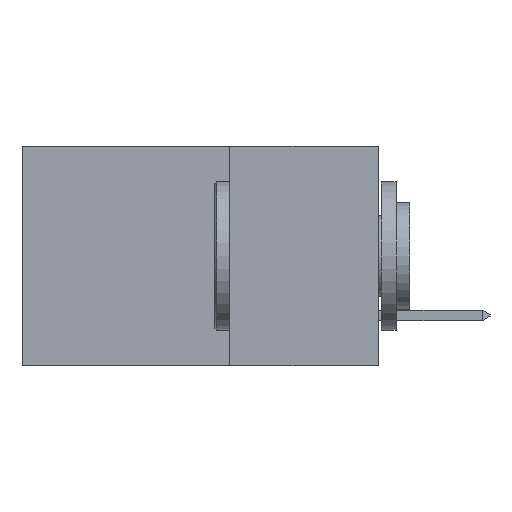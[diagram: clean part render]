
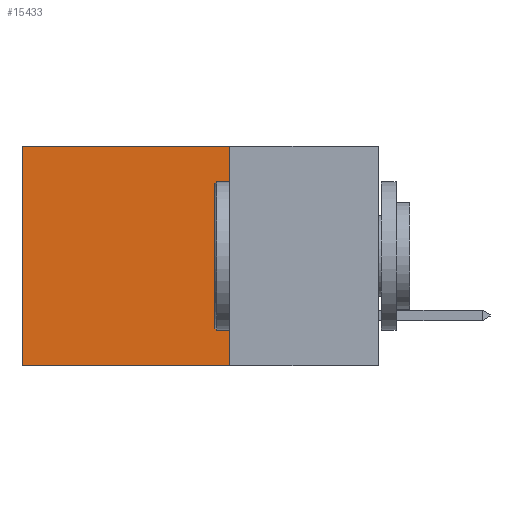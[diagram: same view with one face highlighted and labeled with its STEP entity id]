
A CAD part, left-side view. The second image highlights one B-rep face of the part: STEP entity #15433.
In plain terms, the highlighted planar face has unit normal (-1, 0, 0).
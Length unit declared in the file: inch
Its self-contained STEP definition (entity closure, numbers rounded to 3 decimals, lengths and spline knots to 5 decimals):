
#584 = ORIENTED_EDGE ( 'NONE', *, *, #5645, .F. ) ;
#1097 = FACE_OUTER_BOUND ( 'NONE', #2880, .T. ) ;
#1287 = ORIENTED_EDGE ( 'NONE', *, *, #19993, .F. ) ;
#1569 = LINE ( 'NONE', #4928, #19775 ) ;
#2152 = LINE ( 'NONE', #17924, #16239 ) ;
#2165 = CARTESIAN_POINT ( 'NONE',  ( 0.298, 0.25, 0. ) ) ;
#2408 = VECTOR ( 'NONE', #8987, 39.37008 ) ;
#2507 = ORIENTED_EDGE ( 'NONE', *, *, #7538, .T. ) ;
#2880 = EDGE_LOOP ( 'NONE', ( #13797, #584, #1287, #2507 ) ) ;
#3808 = PLANE ( 'NONE',  #9138 ) ;
#3880 = DIRECTION ( 'NONE',  ( 0., 0., -1. ) ) ;
#4108 = DIRECTION ( 'NONE',  ( 0., 1., 0. ) ) ;
#4928 = CARTESIAN_POINT ( 'NONE',  ( 0.298, 0.25, 0. ) ) ;
#5219 = VECTOR ( 'NONE', #4108, 39.37008 ) ;
#5645 = EDGE_CURVE ( 'NONE', #12891, #8686, #14137, .T. ) ;
#7235 = CARTESIAN_POINT ( 'NONE',  ( 0.298, 0.6, -0.37 ) ) ;
#7538 = EDGE_CURVE ( 'NONE', #11624, #19012, #15942, .T. ) ;
#8686 = VERTEX_POINT ( 'NONE', #7235 ) ;
#8987 = DIRECTION ( 'NONE',  ( 0., 1., 0. ) ) ;
#9079 = CARTESIAN_POINT ( 'NONE',  ( 0.298, 0.25, 0. ) ) ;
#9138 = AXIS2_PLACEMENT_3D ( 'NONE', #2165, #14524, #3880 ) ;
#9157 = DIRECTION ( 'NONE',  ( 0., 0., -1. ) ) ;
#10716 = CARTESIAN_POINT ( 'NONE',  ( 0.298, 0.25, -0.37 ) ) ;
#11254 = CARTESIAN_POINT ( 'NONE',  ( 0.298, 0.25, -0.37 ) ) ;
#11624 = VERTEX_POINT ( 'NONE', #9079 ) ;
#12118 = DIRECTION ( 'NONE',  ( 0., 0., -1. ) ) ;
#12891 = VERTEX_POINT ( 'NONE', #10716 ) ;
#13797 = ORIENTED_EDGE ( 'NONE', *, *, #19052, .T. ) ;
#14137 = LINE ( 'NONE', #11254, #5219 ) ;
#14524 = DIRECTION ( 'NONE',  ( 1., 0., 0. ) ) ;
#15433 = ADVANCED_FACE ( 'NONE', ( #1097 ), #3808, .F. ) ;
#15942 = LINE ( 'NONE', #19494, #2408 ) ;
#16239 = VECTOR ( 'NONE', #9157, 39.37008 ) ;
#17924 = CARTESIAN_POINT ( 'NONE',  ( 0.298, 0.6, 0. ) ) ;
#19012 = VERTEX_POINT ( 'NONE', #19596 ) ;
#19052 = EDGE_CURVE ( 'NONE', #19012, #8686, #2152, .T. ) ;
#19494 = CARTESIAN_POINT ( 'NONE',  ( 0.298, 0.25, 0. ) ) ;
#19596 = CARTESIAN_POINT ( 'NONE',  ( 0.298, 0.6, 0. ) ) ;
#19775 = VECTOR ( 'NONE', #12118, 39.37008 ) ;
#19993 = EDGE_CURVE ( 'NONE', #11624, #12891, #1569, .T. ) ;
